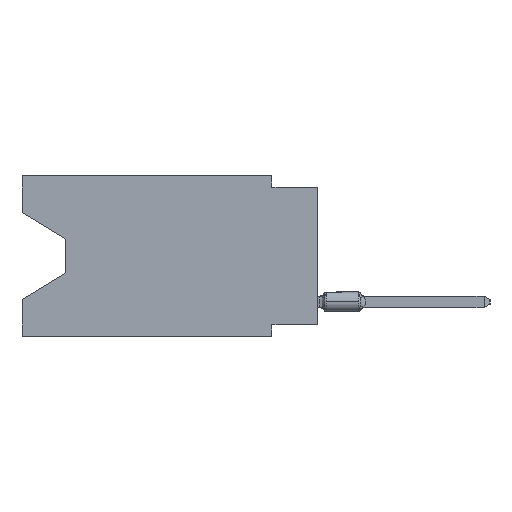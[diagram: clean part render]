
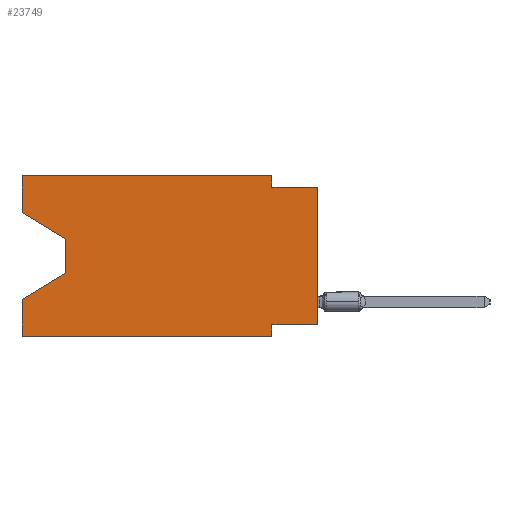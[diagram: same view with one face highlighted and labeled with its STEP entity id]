
A CAD part, left-side view. The second image highlights one B-rep face of the part: STEP entity #23749.
In plain terms, the highlighted planar face has unit normal (-1, 0, 0).
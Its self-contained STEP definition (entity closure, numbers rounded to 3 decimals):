
#203 = CARTESIAN_POINT ( 'NONE',  ( 0., 16.383, -2.038 ) ) ;
#1413 = EDGE_CURVE ( 'NONE', #11246, #11117, #9779, .T. ) ;
#1585 = LINE ( 'NONE', #20650, #21159 ) ;
#1969 = DIRECTION ( 'NONE',  ( 0., -1., 0. ) ) ;
#2591 = EDGE_CURVE ( 'NONE', #21876, #11370, #25462, .T. ) ;
#2947 = ORIENTED_EDGE ( 'NONE', *, *, #8127, .F. ) ;
#3189 = CARTESIAN_POINT ( 'NONE',  ( 0., 0., -8.255 ) ) ;
#3427 = ORIENTED_EDGE ( 'NONE', *, *, #23894, .T. ) ;
#3837 = LINE ( 'NONE', #6178, #7524 ) ;
#3934 = CARTESIAN_POINT ( 'NONE',  ( 0., 0., -0.635 ) ) ;
#3953 = ORIENTED_EDGE ( 'NONE', *, *, #17218, .T. ) ;
#4027 = LINE ( 'NONE', #203, #18768 ) ;
#4508 = EDGE_CURVE ( 'NONE', #21876, #11246, #15603, .T. ) ;
#4666 = VECTOR ( 'NONE', #11230, 1000. ) ;
#4767 = LINE ( 'NONE', #20717, #25155 ) ;
#5610 = CARTESIAN_POINT ( 'NONE',  ( 0., 2.54, 0. ) ) ;
#5689 = DIRECTION ( 'NONE',  ( 0., 1., 0. ) ) ;
#5874 = VECTOR ( 'NONE', #17753, 1000. ) ;
#5879 = VECTOR ( 'NONE', #13172, 1000. ) ;
#5994 = LINE ( 'NONE', #5610, #12962 ) ;
#5997 = CARTESIAN_POINT ( 'NONE',  ( 0., 16.383, -8.89 ) ) ;
#6178 = CARTESIAN_POINT ( 'NONE',  ( 0., 16.383, 0. ) ) ;
#6257 = LINE ( 'NONE', #24401, #23261 ) ;
#6496 = CARTESIAN_POINT ( 'NONE',  ( 0., 16.383, -6.852 ) ) ;
#6904 = ORIENTED_EDGE ( 'NONE', *, *, #11954, .F. ) ;
#7203 = ORIENTED_EDGE ( 'NONE', *, *, #2591, .T. ) ;
#7524 = VECTOR ( 'NONE', #11809, 1000. ) ;
#7823 = AXIS2_PLACEMENT_3D ( 'NONE', #15802, #19882, #25342 ) ;
#8092 = CARTESIAN_POINT ( 'NONE',  ( 0., 16.383, 0. ) ) ;
#8127 = EDGE_CURVE ( 'NONE', #20895, #11370, #19902, .T. ) ;
#8530 = ORIENTED_EDGE ( 'NONE', *, *, #1413, .F. ) ;
#8970 = CARTESIAN_POINT ( 'NONE',  ( 0., 13.97, -3.505 ) ) ;
#9125 = VERTEX_POINT ( 'NONE', #15519 ) ;
#9269 = EDGE_CURVE ( 'NONE', #23466, #16799, #4027, .T. ) ;
#9779 = LINE ( 'NONE', #25703, #5874 ) ;
#9889 = EDGE_LOOP ( 'NONE', ( #24331, #12817, #3953, #19474, #3427, #8530, #18005, #7203, #2947, #6904, #16687, #18477 ) ) ;
#10553 = VERTEX_POINT ( 'NONE', #5997 ) ;
#11049 = EDGE_CURVE ( 'NONE', #23466, #15875, #3837, .T. ) ;
#11117 = VERTEX_POINT ( 'NONE', #14639 ) ;
#11230 = DIRECTION ( 'NONE',  ( 0., 0., 1. ) ) ;
#11246 = VERTEX_POINT ( 'NONE', #19105 ) ;
#11370 = VERTEX_POINT ( 'NONE', #21594 ) ;
#11786 = EDGE_CURVE ( 'NONE', #16799, #16545, #15004, .T. ) ;
#11809 = DIRECTION ( 'NONE',  ( 0., 0., 1. ) ) ;
#11954 = EDGE_CURVE ( 'NONE', #9125, #20895, #5994, .T. ) ;
#12002 = DIRECTION ( 'NONE',  ( 0., -0.855, -0.519 ) ) ;
#12413 = CARTESIAN_POINT ( 'NONE',  ( 0., 16.383, -2.038 ) ) ;
#12817 = ORIENTED_EDGE ( 'NONE', *, *, #11786, .T. ) ;
#12867 = VECTOR ( 'NONE', #1969, 1000. ) ;
#12962 = VECTOR ( 'NONE', #25845, 1000. ) ;
#13110 = CARTESIAN_POINT ( 'NONE',  ( 0., 13.97, -5.385 ) ) ;
#13172 = DIRECTION ( 'NONE',  ( 0., 0., -1. ) ) ;
#13457 = PLANE ( 'NONE',  #7823 ) ;
#14591 = DIRECTION ( 'NONE',  ( 0., -1., 0. ) ) ;
#14639 = CARTESIAN_POINT ( 'NONE',  ( 0., 2.54, -8.89 ) ) ;
#15004 = LINE ( 'NONE', #21018, #5879 ) ;
#15519 = CARTESIAN_POINT ( 'NONE',  ( 0., 2.54, 0. ) ) ;
#15528 = CARTESIAN_POINT ( 'NONE',  ( 0., 0., 0. ) ) ;
#15603 = LINE ( 'NONE', #3189, #24372 ) ;
#15802 = CARTESIAN_POINT ( 'NONE',  ( 0., 16.383, 0. ) ) ;
#15875 = VERTEX_POINT ( 'NONE', #8092 ) ;
#16003 = VERTEX_POINT ( 'NONE', #6496 ) ;
#16545 = VERTEX_POINT ( 'NONE', #22668 ) ;
#16547 = EDGE_CURVE ( 'NONE', #15875, #9125, #4767, .T. ) ;
#16687 = ORIENTED_EDGE ( 'NONE', *, *, #16547, .F. ) ;
#16799 = VERTEX_POINT ( 'NONE', #8970 ) ;
#17218 = EDGE_CURVE ( 'NONE', #16545, #16003, #19142, .T. ) ;
#17753 = DIRECTION ( 'NONE',  ( 0., 0., -1. ) ) ;
#17777 = FACE_OUTER_BOUND ( 'NONE', #9889, .T. ) ;
#18005 = ORIENTED_EDGE ( 'NONE', *, *, #4508, .F. ) ;
#18477 = ORIENTED_EDGE ( 'NONE', *, *, #11049, .F. ) ;
#18725 = CARTESIAN_POINT ( 'NONE',  ( 0., 0., -8.255 ) ) ;
#18745 = DIRECTION ( 'NONE',  ( 0., 0.855, -0.519 ) ) ;
#18764 = DIRECTION ( 'NONE',  ( 0., -1., 0. ) ) ;
#18768 = VECTOR ( 'NONE', #12002, 1000. ) ;
#19105 = CARTESIAN_POINT ( 'NONE',  ( 0., 2.54, -8.255 ) ) ;
#19142 = LINE ( 'NONE', #13110, #22276 ) ;
#19474 = ORIENTED_EDGE ( 'NONE', *, *, #23321, .F. ) ;
#19882 = DIRECTION ( 'NONE',  ( 1., 0., 0. ) ) ;
#19902 = LINE ( 'NONE', #3934, #12867 ) ;
#20281 = DIRECTION ( 'NONE',  ( 0., 0., 1. ) ) ;
#20650 = CARTESIAN_POINT ( 'NONE',  ( 0., 16.383, 0. ) ) ;
#20717 = CARTESIAN_POINT ( 'NONE',  ( 0., 16.383, 0. ) ) ;
#20895 = VERTEX_POINT ( 'NONE', #21605 ) ;
#21018 = CARTESIAN_POINT ( 'NONE',  ( 0., 13.97, -3.505 ) ) ;
#21159 = VECTOR ( 'NONE', #20281, 1000. ) ;
#21594 = CARTESIAN_POINT ( 'NONE',  ( 0., 0., -0.635 ) ) ;
#21605 = CARTESIAN_POINT ( 'NONE',  ( 0., 2.54, -0.635 ) ) ;
#21876 = VERTEX_POINT ( 'NONE', #18725 ) ;
#22276 = VECTOR ( 'NONE', #18745, 1000. ) ;
#22668 = CARTESIAN_POINT ( 'NONE',  ( 0., 13.97, -5.385 ) ) ;
#23261 = VECTOR ( 'NONE', #14591, 1000. ) ;
#23321 = EDGE_CURVE ( 'NONE', #10553, #16003, #1585, .T. ) ;
#23466 = VERTEX_POINT ( 'NONE', #12413 ) ;
#23749 = ADVANCED_FACE ( 'NONE', ( #17777 ), #13457, .F. ) ;
#23894 = EDGE_CURVE ( 'NONE', #10553, #11117, #6257, .T. ) ;
#24331 = ORIENTED_EDGE ( 'NONE', *, *, #9269, .T. ) ;
#24372 = VECTOR ( 'NONE', #5689, 1000. ) ;
#24401 = CARTESIAN_POINT ( 'NONE',  ( 0., 16.383, -8.89 ) ) ;
#25155 = VECTOR ( 'NONE', #18764, 1000. ) ;
#25342 = DIRECTION ( 'NONE',  ( 0., 0., -1. ) ) ;
#25462 = LINE ( 'NONE', #15528, #4666 ) ;
#25703 = CARTESIAN_POINT ( 'NONE',  ( 0., 2.54, -8.89 ) ) ;
#25845 = DIRECTION ( 'NONE',  ( 0., 0., -1. ) ) ;
